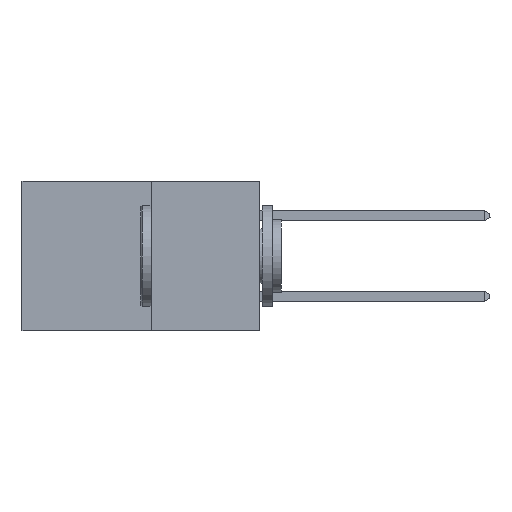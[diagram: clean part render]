
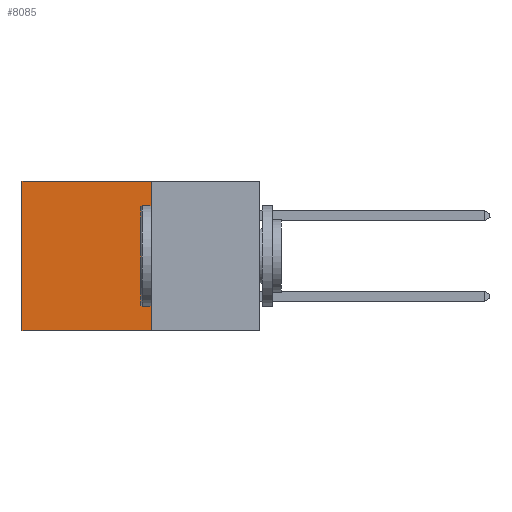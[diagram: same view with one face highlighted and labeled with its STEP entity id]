
A CAD part, left-side view. The second image highlights one B-rep face of the part: STEP entity #8085.
In plain terms, the highlighted planar face has unit normal (-1, 0, 0).
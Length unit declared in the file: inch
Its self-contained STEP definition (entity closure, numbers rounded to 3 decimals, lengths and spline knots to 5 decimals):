
#188 = FACE_OUTER_BOUND ( 'NONE', #19182, .T. ) ;
#1398 = PLANE ( 'NONE',  #19382 ) ;
#2672 = VECTOR ( 'NONE', #4539, 39.37008 ) ;
#3199 = DIRECTION ( 'NONE',  ( 0., 1., 0. ) ) ;
#4539 = DIRECTION ( 'NONE',  ( 0., 0., -1. ) ) ;
#4569 = EDGE_CURVE ( 'NONE', #16884, #14543, #15766, .T. ) ;
#5391 = ORIENTED_EDGE ( 'NONE', *, *, #30151, .F. ) ;
#6372 = CARTESIAN_POINT ( 'NONE',  ( 0.277, 0.27, -0.37 ) ) ;
#8085 = ADVANCED_FACE ( 'NONE', ( #188 ), #1398, .F. ) ;
#8448 = ORIENTED_EDGE ( 'NONE', *, *, #4569, .F. ) ;
#9305 = VERTEX_POINT ( 'NONE', #13079 ) ;
#9647 = EDGE_CURVE ( 'NONE', #15847, #9305, #26594, .T. ) ;
#10457 = CARTESIAN_POINT ( 'NONE',  ( 0.277, 0.27, -0.37 ) ) ;
#10535 = CARTESIAN_POINT ( 'NONE',  ( 0.277, 0.27, -0.37 ) ) ;
#11689 = CARTESIAN_POINT ( 'NONE',  ( 0.277, 0.59, -0.37 ) ) ;
#11800 = DIRECTION ( 'NONE',  ( 0., 0., -1. ) ) ;
#13079 = CARTESIAN_POINT ( 'NONE',  ( 0.277, 0.59, -0.37 ) ) ;
#13232 = CARTESIAN_POINT ( 'NONE',  ( 0.277, 0.27, 0. ) ) ;
#13774 = DIRECTION ( 'NONE',  ( 1., 0., 0. ) ) ;
#14252 = ORIENTED_EDGE ( 'NONE', *, *, #15092, .T. ) ;
#14466 = LINE ( 'NONE', #13232, #20252 ) ;
#14543 = VERTEX_POINT ( 'NONE', #25922 ) ;
#15092 = EDGE_CURVE ( 'NONE', #16884, #15847, #14466, .T. ) ;
#15766 = LINE ( 'NONE', #10457, #2672 ) ;
#15847 = VERTEX_POINT ( 'NONE', #29319 ) ;
#16884 = VERTEX_POINT ( 'NONE', #22936 ) ;
#18160 = VECTOR ( 'NONE', #3199, 39.37008 ) ;
#19182 = EDGE_LOOP ( 'NONE', ( #19490, #5391, #8448, #14252 ) ) ;
#19382 = AXIS2_PLACEMENT_3D ( 'NONE', #6372, #13774, #30851 ) ;
#19490 = ORIENTED_EDGE ( 'NONE', *, *, #9647, .T. ) ;
#20113 = VECTOR ( 'NONE', #11800, 39.37008 ) ;
#20252 = VECTOR ( 'NONE', #25562, 39.37008 ) ;
#22936 = CARTESIAN_POINT ( 'NONE',  ( 0.277, 0.27, 0. ) ) ;
#24694 = LINE ( 'NONE', #10535, #18160 ) ;
#25562 = DIRECTION ( 'NONE',  ( 0., 1., 0. ) ) ;
#25922 = CARTESIAN_POINT ( 'NONE',  ( 0.277, 0.27, -0.37 ) ) ;
#26594 = LINE ( 'NONE', #11689, #20113 ) ;
#29319 = CARTESIAN_POINT ( 'NONE',  ( 0.277, 0.59, 0. ) ) ;
#30151 = EDGE_CURVE ( 'NONE', #14543, #9305, #24694, .T. ) ;
#30851 = DIRECTION ( 'NONE',  ( 0., 0., -1. ) ) ;
